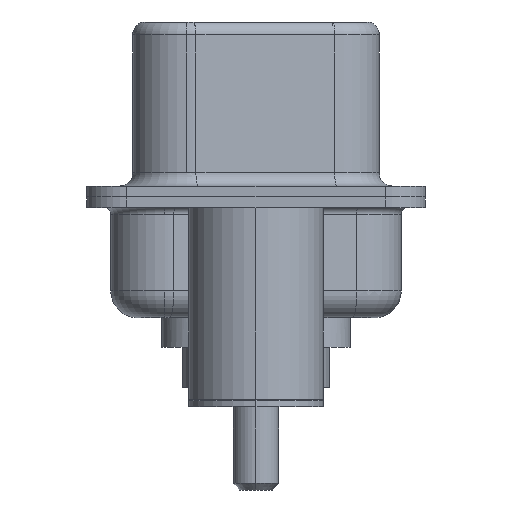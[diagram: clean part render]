
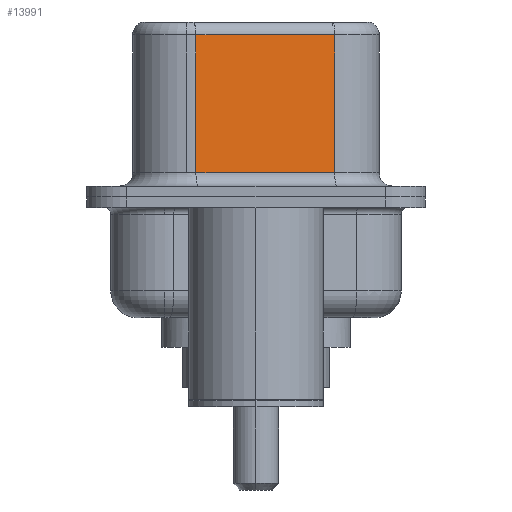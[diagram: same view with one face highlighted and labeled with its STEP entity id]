
A CAD part, left-side view. The second image highlights one B-rep face of the part: STEP entity #13991.
In plain terms, the highlighted planar face has unit normal (-0.985, -0.174, 0).
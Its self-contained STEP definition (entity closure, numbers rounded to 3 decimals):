
#69 = ORIENTED_EDGE ( 'NONE', *, *, #4109, .F. ) ;
#453 = LINE ( 'NONE', #11739, #13921 ) ;
#903 = CARTESIAN_POINT ( 'NONE',  ( 4.58, -2.927, 6.52 ) ) ;
#1718 = DIRECTION ( 'NONE',  ( 0.985, 0.174, 0. ) ) ;
#2387 = LINE ( 'NONE', #903, #12711 ) ;
#3080 = DIRECTION ( 'NONE',  ( -0.174, 0.985, 0. ) ) ;
#4109 = EDGE_CURVE ( 'NONE', #6591, #7142, #2387, .T. ) ;
#4214 = ORIENTED_EDGE ( 'NONE', *, *, #17797, .T. ) ;
#4345 = CARTESIAN_POINT ( 'NONE',  ( 3.67, 2.233, 6.52 ) ) ;
#4821 = CARTESIAN_POINT ( 'NONE',  ( 4.58, -2.927, 6.52 ) ) ;
#5111 = ORIENTED_EDGE ( 'NONE', *, *, #17642, .T. ) ;
#6591 = VERTEX_POINT ( 'NONE', #13132 ) ;
#7142 = VERTEX_POINT ( 'NONE', #19332 ) ;
#7516 = LINE ( 'NONE', #4345, #12206 ) ;
#7536 = DIRECTION ( 'NONE',  ( 0., 0., -1. ) ) ;
#8501 = CARTESIAN_POINT ( 'NONE',  ( 4.58, -2.927, 0.9 ) ) ;
#8767 = CARTESIAN_POINT ( 'NONE',  ( 3.67, 2.233, 6.02 ) ) ;
#8801 = DIRECTION ( 'NONE',  ( 0., 0., -1. ) ) ;
#8952 = VERTEX_POINT ( 'NONE', #8767 ) ;
#9446 = PLANE ( 'NONE',  #19466 ) ;
#9547 = VERTEX_POINT ( 'NONE', #14370 ) ;
#10371 = DIRECTION ( 'NONE',  ( -0.174, 0.985, 0. ) ) ;
#11167 = ORIENTED_EDGE ( 'NONE', *, *, #11811, .T. ) ;
#11739 = CARTESIAN_POINT ( 'NONE',  ( 4.58, -2.927, 6.02 ) ) ;
#11811 = EDGE_CURVE ( 'NONE', #8952, #9547, #7516, .T. ) ;
#12206 = VECTOR ( 'NONE', #7536, 1000. ) ;
#12711 = VECTOR ( 'NONE', #8801, 1000. ) ;
#12995 = EDGE_LOOP ( 'NONE', ( #69, #4214, #11167, #5111 ) ) ;
#13132 = CARTESIAN_POINT ( 'NONE',  ( 4.58, -2.927, 6.02 ) ) ;
#13921 = VECTOR ( 'NONE', #10371, 1000. ) ;
#13991 = ADVANCED_FACE ( 'NONE', ( #15271 ), #9446, .F. ) ;
#14370 = CARTESIAN_POINT ( 'NONE',  ( 3.67, 2.233, 0.9 ) ) ;
#14886 = LINE ( 'NONE', #8501, #18110 ) ;
#15271 = FACE_OUTER_BOUND ( 'NONE', #12995, .T. ) ;
#16304 = DIRECTION ( 'NONE',  ( 0.174, -0.985, 0. ) ) ;
#17642 = EDGE_CURVE ( 'NONE', #9547, #7142, #14886, .T. ) ;
#17797 = EDGE_CURVE ( 'NONE', #6591, #8952, #453, .T. ) ;
#18110 = VECTOR ( 'NONE', #16304, 1000. ) ;
#19332 = CARTESIAN_POINT ( 'NONE',  ( 4.58, -2.927, 0.9 ) ) ;
#19466 = AXIS2_PLACEMENT_3D ( 'NONE', #4821, #1718, #3080 ) ;
